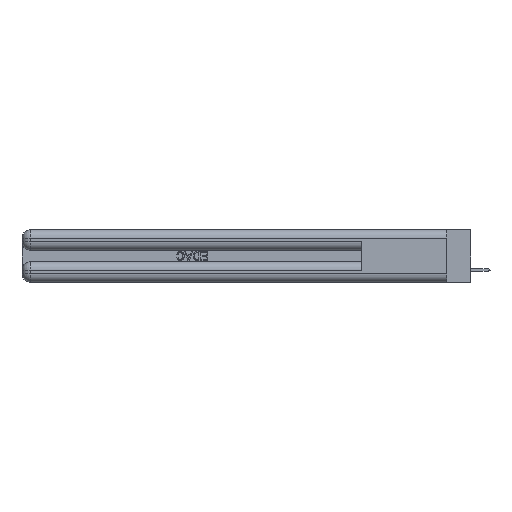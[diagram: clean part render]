
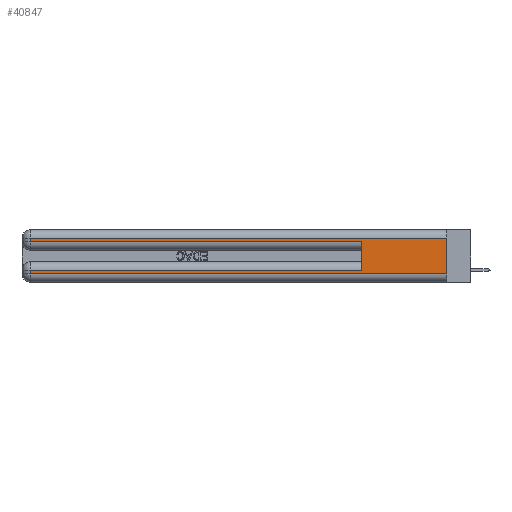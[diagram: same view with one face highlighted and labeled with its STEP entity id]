
A CAD part, left-side view. The second image highlights one B-rep face of the part: STEP entity #40847.
In plain terms, the highlighted planar face has unit normal (-1, 0, 0).
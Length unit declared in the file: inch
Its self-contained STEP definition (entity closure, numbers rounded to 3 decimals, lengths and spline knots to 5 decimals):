
#221 = EDGE_CURVE ( 'NONE', #31679, #21618, #9348, .T. ) ;
#864 = CARTESIAN_POINT ( 'NONE',  ( 0., 0., 0.37 ) ) ;
#1259 = LINE ( 'NONE', #44568, #35877 ) ;
#1447 = VERTEX_POINT ( 'NONE', #42973 ) ;
#2819 = EDGE_LOOP ( 'NONE', ( #40658, #25668, #10682, #31743, #30619, #32463, #16538, #31273 ) ) ;
#2822 = VERTEX_POINT ( 'NONE', #8779 ) ;
#3266 = DIRECTION ( 'NONE',  ( 0., 0., -1. ) ) ;
#4445 = VECTOR ( 'NONE', #25336, 39.37008 ) ;
#4939 = VERTEX_POINT ( 'NONE', #33777 ) ;
#5299 = EDGE_CURVE ( 'NONE', #22451, #1447, #39595, .T. ) ;
#7850 = VERTEX_POINT ( 'NONE', #17570 ) ;
#7948 = DIRECTION ( 'NONE',  ( 0., 1., 0. ) ) ;
#8134 = DIRECTION ( 'NONE',  ( 0., 0., -1. ) ) ;
#8779 = CARTESIAN_POINT ( 'NONE',  ( 0., 2.94, 0.085 ) ) ;
#9348 = LINE ( 'NONE', #37902, #14041 ) ;
#10682 = ORIENTED_EDGE ( 'NONE', *, *, #24063, .T. ) ;
#11677 = CARTESIAN_POINT ( 'NONE',  ( 0., 0., 0.085 ) ) ;
#14041 = VECTOR ( 'NONE', #20831, 39.37008 ) ;
#14287 = CARTESIAN_POINT ( 'NONE',  ( 0., 2.94, 0.37 ) ) ;
#15106 = VECTOR ( 'NONE', #45535, 39.37008 ) ;
#15882 = LINE ( 'NONE', #11677, #40887 ) ;
#16538 = ORIENTED_EDGE ( 'NONE', *, *, #24130, .T. ) ;
#17459 = EDGE_CURVE ( 'NONE', #7850, #1447, #20560, .T. ) ;
#17570 = CARTESIAN_POINT ( 'NONE',  ( 0., 2.94, 0.06 ) ) ;
#19362 = EDGE_CURVE ( 'NONE', #4939, #21618, #1259, .T. ) ;
#19606 = VECTOR ( 'NONE', #22242, 39.37008 ) ;
#20560 = LINE ( 'NONE', #42063, #40211 ) ;
#20831 = DIRECTION ( 'NONE',  ( 0., -1., 0. ) ) ;
#21618 = VERTEX_POINT ( 'NONE', #26363 ) ;
#21715 = EDGE_CURVE ( 'NONE', #22451, #38535, #23999, .T. ) ;
#21835 = CARTESIAN_POINT ( 'NONE',  ( 0., 2.94, 0.285 ) ) ;
#22242 = DIRECTION ( 'NONE',  ( 0., 0., -1. ) ) ;
#22451 = VERTEX_POINT ( 'NONE', #37077 ) ;
#22464 = LINE ( 'NONE', #26681, #19606 ) ;
#22636 = DIRECTION ( 'NONE',  ( 1., 0., 0. ) ) ;
#23260 = DIRECTION ( 'NONE',  ( 0., 0., 1. ) ) ;
#23999 = LINE ( 'NONE', #34296, #15106 ) ;
#24063 = EDGE_CURVE ( 'NONE', #38535, #31679, #24830, .T. ) ;
#24130 = EDGE_CURVE ( 'NONE', #2822, #7850, #22464, .T. ) ;
#24830 = LINE ( 'NONE', #14287, #24872 ) ;
#24872 = VECTOR ( 'NONE', #3266, 39.37008 ) ;
#25336 = DIRECTION ( 'NONE',  ( 0., 0., -1. ) ) ;
#25668 = ORIENTED_EDGE ( 'NONE', *, *, #21715, .T. ) ;
#26363 = CARTESIAN_POINT ( 'NONE',  ( 0., 0.6, 0.285 ) ) ;
#26681 = CARTESIAN_POINT ( 'NONE',  ( 0., 2.94, 0.37 ) ) ;
#29532 = CARTESIAN_POINT ( 'NONE',  ( 0., 2.94, 0.31 ) ) ;
#30111 = FACE_OUTER_BOUND ( 'NONE', #2819, .T. ) ;
#30619 = ORIENTED_EDGE ( 'NONE', *, *, #19362, .F. ) ;
#31273 = ORIENTED_EDGE ( 'NONE', *, *, #17459, .T. ) ;
#31679 = VERTEX_POINT ( 'NONE', #21835 ) ;
#31743 = ORIENTED_EDGE ( 'NONE', *, *, #221, .T. ) ;
#32463 = ORIENTED_EDGE ( 'NONE', *, *, #37283, .T. ) ;
#33777 = CARTESIAN_POINT ( 'NONE',  ( 0., 0.6, 0.085 ) ) ;
#34296 = CARTESIAN_POINT ( 'NONE',  ( 0., 0., 0.31 ) ) ;
#35877 = VECTOR ( 'NONE', #23260, 39.37008 ) ;
#36326 = CARTESIAN_POINT ( 'NONE',  ( 0., 0., 0.37 ) ) ;
#37077 = CARTESIAN_POINT ( 'NONE',  ( 0., 0., 0.31 ) ) ;
#37283 = EDGE_CURVE ( 'NONE', #4939, #2822, #15882, .T. ) ;
#37902 = CARTESIAN_POINT ( 'NONE',  ( 0., 0., 0.285 ) ) ;
#38008 = AXIS2_PLACEMENT_3D ( 'NONE', #864, #22636, #8134 ) ;
#38093 = DIRECTION ( 'NONE',  ( 0., -1., 0. ) ) ;
#38535 = VERTEX_POINT ( 'NONE', #29532 ) ;
#39595 = LINE ( 'NONE', #36326, #4445 ) ;
#39974 = PLANE ( 'NONE',  #38008 ) ;
#40211 = VECTOR ( 'NONE', #38093, 39.37008 ) ;
#40658 = ORIENTED_EDGE ( 'NONE', *, *, #5299, .F. ) ;
#40847 = ADVANCED_FACE ( 'NONE', ( #30111 ), #39974, .F. ) ;
#40887 = VECTOR ( 'NONE', #7948, 39.37008 ) ;
#42063 = CARTESIAN_POINT ( 'NONE',  ( 0., 0., 0.06 ) ) ;
#42973 = CARTESIAN_POINT ( 'NONE',  ( 0., 0., 0.06 ) ) ;
#44568 = CARTESIAN_POINT ( 'NONE',  ( 0., 0.6, 0.145 ) ) ;
#45535 = DIRECTION ( 'NONE',  ( 0., 1., 0. ) ) ;
